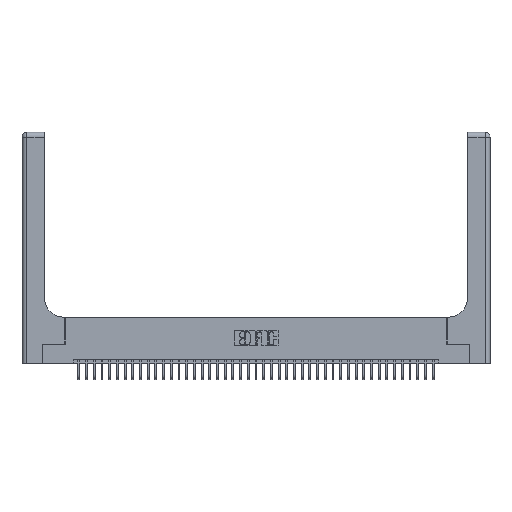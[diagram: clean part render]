
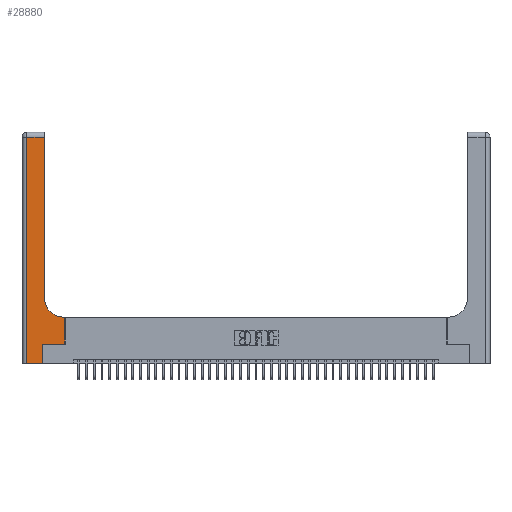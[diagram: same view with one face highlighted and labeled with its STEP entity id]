
A CAD part, top view. The second image highlights one B-rep face of the part: STEP entity #28880.
In plain terms, the highlighted planar face has unit normal (0, 0, 1).
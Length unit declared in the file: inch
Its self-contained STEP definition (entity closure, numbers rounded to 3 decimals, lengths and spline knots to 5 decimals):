
#691 = DIRECTION ( 'NONE',  ( 0., 0., -1. ) ) ;
#1063 = VECTOR ( 'NONE', #6227, 39.37008 ) ;
#1805 = CARTESIAN_POINT ( 'NONE',  ( 0.06, 0., 0.37 ) ) ;
#2603 = DIRECTION ( 'NONE',  ( -1., 0., 0. ) ) ;
#2637 = FACE_OUTER_BOUND ( 'NONE', #19499, .T. ) ;
#2809 = CARTESIAN_POINT ( 'NONE',  ( 0.5585, 0.25, 0.37 ) ) ;
#4025 = DIRECTION ( 'NONE',  ( 1., 0., 0. ) ) ;
#4867 = VECTOR ( 'NONE', #39955, 39.37008 ) ;
#5395 = EDGE_CURVE ( 'NONE', #41188, #24720, #35540, .T. ) ;
#5442 = EDGE_CURVE ( 'NONE', #33726, #7986, #42361, .T. ) ;
#6227 = DIRECTION ( 'NONE',  ( 0., 1., 0. ) ) ;
#6944 = ORIENTED_EDGE ( 'NONE', *, *, #14624, .T. ) ;
#7867 = LINE ( 'NONE', #15621, #33197 ) ;
#7986 = VERTEX_POINT ( 'NONE', #31735 ) ;
#10738 = ORIENTED_EDGE ( 'NONE', *, *, #37323, .T. ) ;
#11757 = VECTOR ( 'NONE', #16543, 39.37008 ) ;
#11825 = AXIS2_PLACEMENT_3D ( 'NONE', #20648, #691, #23937 ) ;
#12503 = VERTEX_POINT ( 'NONE', #40128 ) ;
#13238 = CARTESIAN_POINT ( 'NONE',  ( 0.2915, 3., 0.37 ) ) ;
#13395 = CARTESIAN_POINT ( 'NONE',  ( 0.2915, 0.6, 0.37 ) ) ;
#14624 = EDGE_CURVE ( 'NONE', #7986, #41003, #37484, .T. ) ;
#15055 = ORIENTED_EDGE ( 'NONE', *, *, #5395, .T. ) ;
#15589 = VERTEX_POINT ( 'NONE', #27821 ) ;
#15621 = CARTESIAN_POINT ( 'NONE',  ( 0.06, 3., 0.37 ) ) ;
#15839 = LINE ( 'NONE', #13395, #4867 ) ;
#15901 = VECTOR ( 'NONE', #29169, 39.37008 ) ;
#16543 = DIRECTION ( 'NONE',  ( -1., 0., 0. ) ) ;
#17530 = VECTOR ( 'NONE', #32995, 39.37008 ) ;
#17593 = DIRECTION ( 'NONE',  ( 1., 0., 0. ) ) ;
#17667 = ORIENTED_EDGE ( 'NONE', *, *, #39977, .T. ) ;
#18665 = EDGE_CURVE ( 'NONE', #12503, #15589, #39611, .T. ) ;
#19112 = CARTESIAN_POINT ( 'NONE',  ( 0.269, 0., 0.37 ) ) ;
#19499 = EDGE_LOOP ( 'NONE', ( #33789, #10738, #17667, #15055, #29596, #21199, #6944, #39348, #29796 ) ) ;
#20196 = CARTESIAN_POINT ( 'NONE',  ( 0.5585, 0.6, 0.37 ) ) ;
#20514 = LINE ( 'NONE', #32809, #11757 ) ;
#20648 = CARTESIAN_POINT ( 'NONE',  ( 0.5415, 0.85, 0.37 ) ) ;
#21199 = ORIENTED_EDGE ( 'NONE', *, *, #5442, .T. ) ;
#22532 = DIRECTION ( 'NONE',  ( 0., 0., -1. ) ) ;
#23937 = DIRECTION ( 'NONE',  ( 1., 0., 0. ) ) ;
#23947 = VERTEX_POINT ( 'NONE', #31679 ) ;
#24720 = VERTEX_POINT ( 'NONE', #19112 ) ;
#26231 = EDGE_CURVE ( 'NONE', #15589, #23947, #35117, .T. ) ;
#27704 = VECTOR ( 'NONE', #4025, 39.37008 ) ;
#27758 = AXIS2_PLACEMENT_3D ( 'NONE', #42474, #22532, #2603 ) ;
#27821 = CARTESIAN_POINT ( 'NONE',  ( 0.2915, 0.85, 0.37 ) ) ;
#27946 = EDGE_CURVE ( 'NONE', #41003, #12503, #15839, .T. ) ;
#28880 = ADVANCED_FACE ( 'NONE', ( #2637 ), #32317, .F. ) ;
#29169 = DIRECTION ( 'NONE',  ( 0., 1., 0. ) ) ;
#29596 = ORIENTED_EDGE ( 'NONE', *, *, #37218, .T. ) ;
#29796 = ORIENTED_EDGE ( 'NONE', *, *, #18665, .T. ) ;
#31679 = CARTESIAN_POINT ( 'NONE',  ( 0.2915, 2.94, 0.37 ) ) ;
#31735 = CARTESIAN_POINT ( 'NONE',  ( 0.5585, 0.25, 0.37 ) ) ;
#32010 = DIRECTION ( 'NONE',  ( 0., -1., 0. ) ) ;
#32317 = PLANE ( 'NONE',  #27758 ) ;
#32809 = CARTESIAN_POINT ( 'NONE',  ( 0., 2.94, 0.37 ) ) ;
#32995 = DIRECTION ( 'NONE',  ( 0., 1., 0. ) ) ;
#33197 = VECTOR ( 'NONE', #32010, 39.37008 ) ;
#33726 = VERTEX_POINT ( 'NONE', #41332 ) ;
#33757 = CARTESIAN_POINT ( 'NONE',  ( 0., 0., 0.37 ) ) ;
#33789 = ORIENTED_EDGE ( 'NONE', *, *, #26231, .T. ) ;
#33958 = VERTEX_POINT ( 'NONE', #42608 ) ;
#34046 = CARTESIAN_POINT ( 'NONE',  ( 0.269, 0.25, 0.37 ) ) ;
#34483 = VECTOR ( 'NONE', #17593, 39.37008 ) ;
#35117 = LINE ( 'NONE', #13238, #17530 ) ;
#35540 = LINE ( 'NONE', #33757, #27704 ) ;
#35786 = CARTESIAN_POINT ( 'NONE',  ( 0.269, 0., 0.37 ) ) ;
#37218 = EDGE_CURVE ( 'NONE', #24720, #33726, #42379, .T. ) ;
#37323 = EDGE_CURVE ( 'NONE', #23947, #33958, #20514, .T. ) ;
#37484 = LINE ( 'NONE', #2809, #1063 ) ;
#39348 = ORIENTED_EDGE ( 'NONE', *, *, #27946, .T. ) ;
#39611 = CIRCLE ( 'NONE', #11825, 0.25 ) ;
#39955 = DIRECTION ( 'NONE',  ( -1., 0., 0. ) ) ;
#39977 = EDGE_CURVE ( 'NONE', #33958, #41188, #7867, .T. ) ;
#40128 = CARTESIAN_POINT ( 'NONE',  ( 0.5415, 0.6, 0.37 ) ) ;
#41003 = VERTEX_POINT ( 'NONE', #20196 ) ;
#41188 = VERTEX_POINT ( 'NONE', #1805 ) ;
#41332 = CARTESIAN_POINT ( 'NONE',  ( 0.269, 0.25, 0.37 ) ) ;
#42361 = LINE ( 'NONE', #34046, #34483 ) ;
#42379 = LINE ( 'NONE', #35786, #15901 ) ;
#42474 = CARTESIAN_POINT ( 'NONE',  ( 0., 3., 0.37 ) ) ;
#42608 = CARTESIAN_POINT ( 'NONE',  ( 0.06, 2.94, 0.37 ) ) ;
